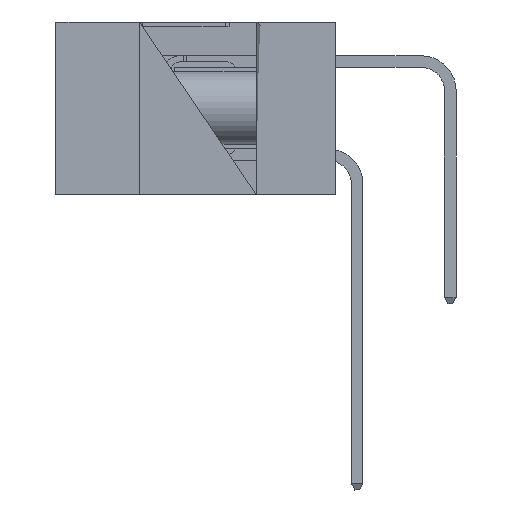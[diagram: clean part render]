
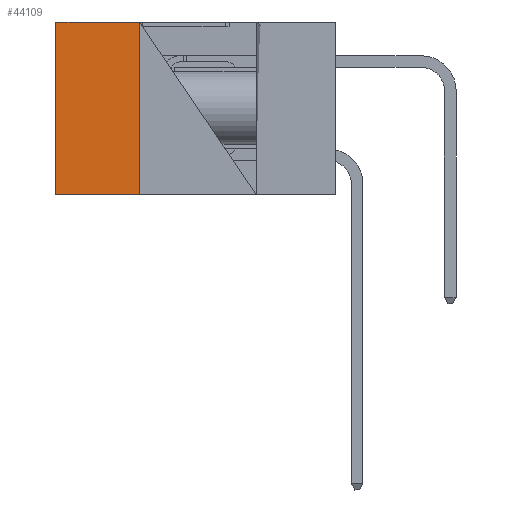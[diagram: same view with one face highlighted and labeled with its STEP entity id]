
A CAD part, left-side view. The second image highlights one B-rep face of the part: STEP entity #44109.
In plain terms, the highlighted planar face has unit normal (-1, 0, 0).
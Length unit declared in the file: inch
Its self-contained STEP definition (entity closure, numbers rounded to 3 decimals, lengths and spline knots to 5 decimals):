
#1297 = EDGE_CURVE ( 'NONE', #33056, #7466, #30991, .T. ) ;
#1505 = EDGE_LOOP ( 'NONE', ( #25232, #9561, #19691, #2506 ) ) ;
#2506 = ORIENTED_EDGE ( 'NONE', *, *, #13312, .T. ) ;
#4539 = DIRECTION ( 'NONE',  ( 1., 0., 0. ) ) ;
#7198 = VERTEX_POINT ( 'NONE', #19936 ) ;
#7466 = VERTEX_POINT ( 'NONE', #13095 ) ;
#8106 = LINE ( 'NONE', #34269, #11270 ) ;
#8192 = VECTOR ( 'NONE', #26495, 39.37008 ) ;
#9561 = ORIENTED_EDGE ( 'NONE', *, *, #19660, .F. ) ;
#11270 = VECTOR ( 'NONE', #30133, 39.37008 ) ;
#13095 = CARTESIAN_POINT ( 'NONE',  ( 0.2875, 0.42, -0.37 ) ) ;
#13312 = EDGE_CURVE ( 'NONE', #33056, #31872, #8106, .T. ) ;
#14310 = CARTESIAN_POINT ( 'NONE',  ( 0.2875, 0.42, -0.37 ) ) ;
#16267 = DIRECTION ( 'NONE',  ( 0., 0., -1. ) ) ;
#17315 = VECTOR ( 'NONE', #18754, 39.37008 ) ;
#18754 = DIRECTION ( 'NONE',  ( 0., 0., -1. ) ) ;
#19660 = EDGE_CURVE ( 'NONE', #7466, #7198, #38319, .T. ) ;
#19691 = ORIENTED_EDGE ( 'NONE', *, *, #1297, .F. ) ;
#19936 = CARTESIAN_POINT ( 'NONE',  ( 0.2875, 0.6, -0.37 ) ) ;
#20629 = CARTESIAN_POINT ( 'NONE',  ( 0.2875, 0.42, 0. ) ) ;
#25232 = ORIENTED_EDGE ( 'NONE', *, *, #31385, .T. ) ;
#26495 = DIRECTION ( 'NONE',  ( 0., 1., 0. ) ) ;
#28392 = VECTOR ( 'NONE', #16267, 39.37008 ) ;
#30133 = DIRECTION ( 'NONE',  ( 0., 1., 0. ) ) ;
#30142 = LINE ( 'NONE', #35113, #17315 ) ;
#30991 = LINE ( 'NONE', #48141, #28392 ) ;
#31385 = EDGE_CURVE ( 'NONE', #31872, #7198, #30142, .T. ) ;
#31872 = VERTEX_POINT ( 'NONE', #43093 ) ;
#32504 = DIRECTION ( 'NONE',  ( 0., 0., -1. ) ) ;
#33056 = VERTEX_POINT ( 'NONE', #37260 ) ;
#34269 = CARTESIAN_POINT ( 'NONE',  ( 0.2875, 0.42, 0. ) ) ;
#35113 = CARTESIAN_POINT ( 'NONE',  ( 0.2875, 0.6, 0. ) ) ;
#37260 = CARTESIAN_POINT ( 'NONE',  ( 0.2875, 0.42, 0. ) ) ;
#38319 = LINE ( 'NONE', #14310, #8192 ) ;
#38847 = AXIS2_PLACEMENT_3D ( 'NONE', #20629, #4539, #32504 ) ;
#43093 = CARTESIAN_POINT ( 'NONE',  ( 0.2875, 0.6, 0. ) ) ;
#44109 = ADVANCED_FACE ( 'NONE', ( #50147 ), #45017, .F. ) ;
#45017 = PLANE ( 'NONE',  #38847 ) ;
#48141 = CARTESIAN_POINT ( 'NONE',  ( 0.2875, 0.42, 0. ) ) ;
#50147 = FACE_OUTER_BOUND ( 'NONE', #1505, .T. ) ;
